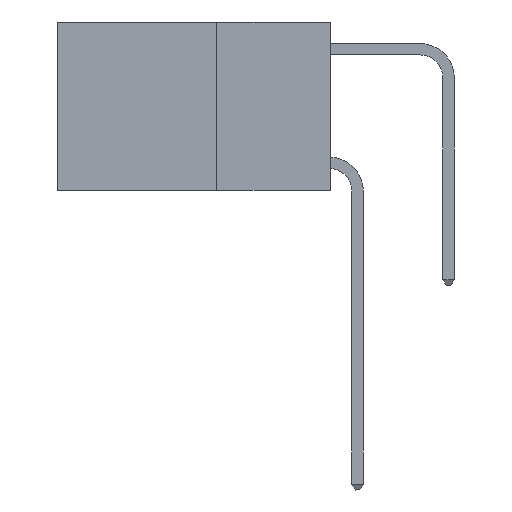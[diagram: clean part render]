
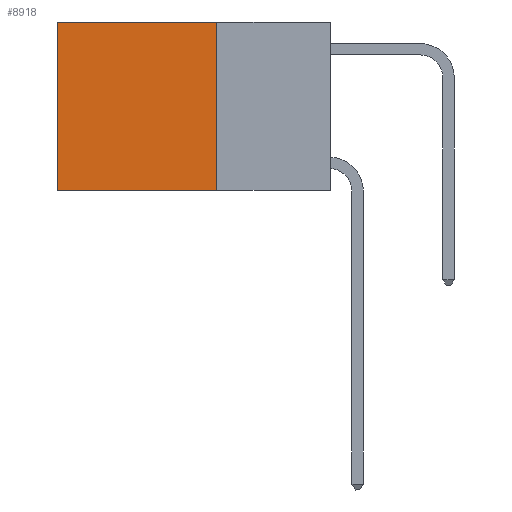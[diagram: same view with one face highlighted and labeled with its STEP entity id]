
A CAD part, left-side view. The second image highlights one B-rep face of the part: STEP entity #8918.
In plain terms, the highlighted planar face has unit normal (-1, 0, 0).
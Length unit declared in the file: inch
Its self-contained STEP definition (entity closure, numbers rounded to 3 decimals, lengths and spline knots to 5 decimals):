
#333 = CARTESIAN_POINT ( 'NONE',  ( 0.2625, 0.25, 0. ) ) ;
#600 = VERTEX_POINT ( 'NONE', #333 ) ;
#875 = LINE ( 'NONE', #5658, #8688 ) ;
#900 = CARTESIAN_POINT ( 'NONE',  ( 0.2625, 0.6, 0. ) ) ;
#1204 = ORIENTED_EDGE ( 'NONE', *, *, #2579, .F. ) ;
#1263 = EDGE_CURVE ( 'NONE', #600, #5809, #875, .T. ) ;
#1441 = DIRECTION ( 'NONE',  ( 0., 1., 0. ) ) ;
#1471 = VECTOR ( 'NONE', #7472, 39.37008 ) ;
#1937 = PLANE ( 'NONE',  #8777 ) ;
#2579 = EDGE_CURVE ( 'NONE', #5809, #10130, #5050, .T. ) ;
#2925 = FACE_OUTER_BOUND ( 'NONE', #3446, .T. ) ;
#2961 = LINE ( 'NONE', #900, #3783 ) ;
#2975 = ORIENTED_EDGE ( 'NONE', *, *, #1263, .F. ) ;
#3446 = EDGE_LOOP ( 'NONE', ( #7012, #1204, #2975, #10806 ) ) ;
#3783 = VECTOR ( 'NONE', #5804, 39.37008 ) ;
#4727 = CARTESIAN_POINT ( 'NONE',  ( 0.2625, 0.6, 0. ) ) ;
#5050 = LINE ( 'NONE', #10862, #9353 ) ;
#5256 = EDGE_CURVE ( 'NONE', #7083, #10130, #2961, .T. ) ;
#5405 = LINE ( 'NONE', #9257, #1471 ) ;
#5658 = CARTESIAN_POINT ( 'NONE',  ( 0.2625, 0.25, 0. ) ) ;
#5804 = DIRECTION ( 'NONE',  ( 0., 0., -1. ) ) ;
#5809 = VERTEX_POINT ( 'NONE', #10674 ) ;
#6721 = CARTESIAN_POINT ( 'NONE',  ( 0.2625, 0.25, 0. ) ) ;
#7012 = ORIENTED_EDGE ( 'NONE', *, *, #5256, .T. ) ;
#7083 = VERTEX_POINT ( 'NONE', #4727 ) ;
#7472 = DIRECTION ( 'NONE',  ( 0., 1., 0. ) ) ;
#8508 = DIRECTION ( 'NONE',  ( 0., 0., -1. ) ) ;
#8562 = DIRECTION ( 'NONE',  ( 1., 0., 0. ) ) ;
#8688 = VECTOR ( 'NONE', #9502, 39.37008 ) ;
#8777 = AXIS2_PLACEMENT_3D ( 'NONE', #6721, #8562, #8508 ) ;
#8918 = ADVANCED_FACE ( 'NONE', ( #2925 ), #1937, .F. ) ;
#9257 = CARTESIAN_POINT ( 'NONE',  ( 0.2625, 0.25, 0. ) ) ;
#9353 = VECTOR ( 'NONE', #1441, 39.37008 ) ;
#9502 = DIRECTION ( 'NONE',  ( 0., 0., -1. ) ) ;
#10130 = VERTEX_POINT ( 'NONE', #11555 ) ;
#10674 = CARTESIAN_POINT ( 'NONE',  ( 0.2625, 0.25, -0.37 ) ) ;
#10806 = ORIENTED_EDGE ( 'NONE', *, *, #11810, .T. ) ;
#10862 = CARTESIAN_POINT ( 'NONE',  ( 0.2625, 0.25, -0.37 ) ) ;
#11555 = CARTESIAN_POINT ( 'NONE',  ( 0.2625, 0.6, -0.37 ) ) ;
#11810 = EDGE_CURVE ( 'NONE', #600, #7083, #5405, .T. ) ;
